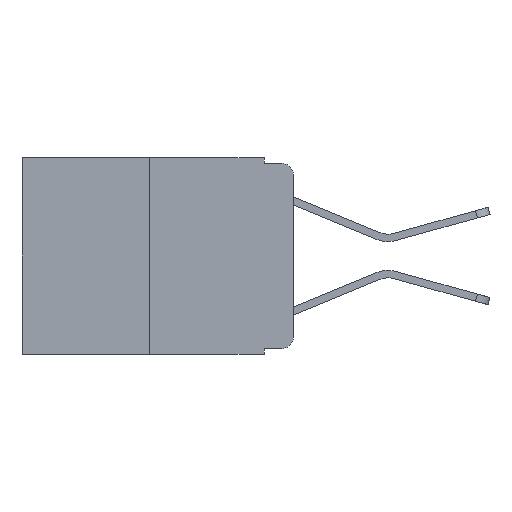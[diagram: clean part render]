
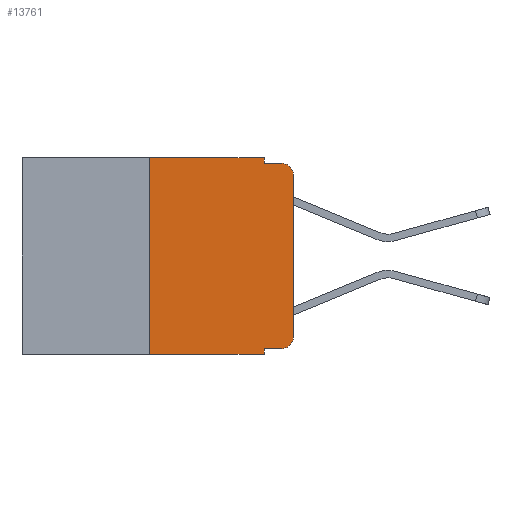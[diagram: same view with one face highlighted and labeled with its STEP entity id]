
A CAD part, left-side view. The second image highlights one B-rep face of the part: STEP entity #13761.
In plain terms, the highlighted planar face has unit normal (-1, 0, 0).
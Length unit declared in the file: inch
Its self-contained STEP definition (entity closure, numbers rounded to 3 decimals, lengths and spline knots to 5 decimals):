
#338 = VERTEX_POINT ( 'NONE', #4138 ) ;
#346 = DIRECTION ( 'NONE',  ( 1., 0., 0. ) ) ;
#349 = DIRECTION ( 'NONE',  ( 0., 0., -1. ) ) ;
#640 = VERTEX_POINT ( 'NONE', #7915 ) ;
#742 = CARTESIAN_POINT ( 'NONE',  ( 0., 0.051, 0. ) ) ;
#946 = VECTOR ( 'NONE', #1736, 39.37008 ) ;
#1036 = DIRECTION ( 'NONE',  ( -1., 0., 0. ) ) ;
#1514 = ORIENTED_EDGE ( 'NONE', *, *, #11581, .F. ) ;
#1736 = DIRECTION ( 'NONE',  ( 0., -1., 0. ) ) ;
#2160 = AXIS2_PLACEMENT_3D ( 'NONE', #17312, #9170, #349 ) ;
#2441 = ORIENTED_EDGE ( 'NONE', *, *, #17806, .F. ) ;
#2626 = LINE ( 'NONE', #14150, #10769 ) ;
#2885 = CARTESIAN_POINT ( 'NONE',  ( 0., 0.25, 0. ) ) ;
#2997 = CIRCLE ( 'NONE', #15039, 0.02 ) ;
#3247 = DIRECTION ( 'NONE',  ( 0., 0., 1. ) ) ;
#3428 = VECTOR ( 'NONE', #4094, 39.37008 ) ;
#3543 = DIRECTION ( 'NONE',  ( 0., 0., -1. ) ) ;
#4094 = DIRECTION ( 'NONE',  ( 0., 0., 1. ) ) ;
#4138 = CARTESIAN_POINT ( 'NONE',  ( 0., 0.02, -0.333 ) ) ;
#4234 = LINE ( 'NONE', #14015, #15026 ) ;
#4665 = AXIS2_PLACEMENT_3D ( 'NONE', #9167, #346, #10566 ) ;
#5112 = LINE ( 'NONE', #17452, #8095 ) ;
#5342 = DIRECTION ( 'NONE',  ( 0., -1., 0. ) ) ;
#5730 = DIRECTION ( 'NONE',  ( 0., 0., -1. ) ) ;
#5823 = LINE ( 'NONE', #17188, #17304 ) ;
#5868 = EDGE_CURVE ( 'NONE', #338, #16558, #2997, .T. ) ;
#6133 = CARTESIAN_POINT ( 'NONE',  ( 0., 0., -0.03 ) ) ;
#6172 = VERTEX_POINT ( 'NONE', #6133 ) ;
#6791 = ORIENTED_EDGE ( 'NONE', *, *, #9722, .F. ) ;
#6834 = EDGE_CURVE ( 'NONE', #640, #338, #14729, .T. ) ;
#6932 = EDGE_LOOP ( 'NONE', ( #8412, #12504, #1514, #13377, #2441, #6791, #10597, #11007, #14686, #11454 ) ) ;
#7082 = FACE_OUTER_BOUND ( 'NONE', #6932, .T. ) ;
#7103 = VERTEX_POINT ( 'NONE', #15554 ) ;
#7323 = LINE ( 'NONE', #12598, #3428 ) ;
#7479 = VERTEX_POINT ( 'NONE', #2885 ) ;
#7915 = CARTESIAN_POINT ( 'NONE',  ( 0., 0.051, -0.333 ) ) ;
#8095 = VECTOR ( 'NONE', #3543, 39.37008 ) ;
#8342 = LINE ( 'NONE', #10417, #946 ) ;
#8412 = ORIENTED_EDGE ( 'NONE', *, *, #13422, .T. ) ;
#8497 = CIRCLE ( 'NONE', #2160, 0.02 ) ;
#8804 = EDGE_CURVE ( 'NONE', #640, #11509, #2626, .T. ) ;
#9085 = CARTESIAN_POINT ( 'NONE',  ( 0., 0.25, -0.343 ) ) ;
#9167 = CARTESIAN_POINT ( 'NONE',  ( 0., 0.473, 0. ) ) ;
#9170 = DIRECTION ( 'NONE',  ( -1., 0., 0. ) ) ;
#9722 = EDGE_CURVE ( 'NONE', #14475, #7479, #5823, .T. ) ;
#9793 = CARTESIAN_POINT ( 'NONE',  ( 0., 0.02, -0.313 ) ) ;
#10417 = CARTESIAN_POINT ( 'NONE',  ( 0., 0.473, 0. ) ) ;
#10566 = DIRECTION ( 'NONE',  ( 0., 0., -1. ) ) ;
#10597 = ORIENTED_EDGE ( 'NONE', *, *, #17569, .T. ) ;
#10663 = EDGE_CURVE ( 'NONE', #13917, #13712, #5112, .T. ) ;
#10688 = LINE ( 'NONE', #14187, #17450 ) ;
#10769 = VECTOR ( 'NONE', #5730, 39.37008 ) ;
#11007 = ORIENTED_EDGE ( 'NONE', *, *, #8804, .F. ) ;
#11169 = DIRECTION ( 'NONE',  ( 0., 0., -1. ) ) ;
#11454 = ORIENTED_EDGE ( 'NONE', *, *, #5868, .T. ) ;
#11509 = VERTEX_POINT ( 'NONE', #14062 ) ;
#11581 = EDGE_CURVE ( 'NONE', #13712, #7103, #10688, .T. ) ;
#11824 = CARTESIAN_POINT ( 'NONE',  ( 0., 0.051, -0.01 ) ) ;
#12185 = CARTESIAN_POINT ( 'NONE',  ( 0., 0., -0.313 ) ) ;
#12482 = EDGE_CURVE ( 'NONE', #6172, #7103, #8497, .T. ) ;
#12504 = ORIENTED_EDGE ( 'NONE', *, *, #12482, .T. ) ;
#12598 = CARTESIAN_POINT ( 'NONE',  ( 0., 0., 0. ) ) ;
#13377 = ORIENTED_EDGE ( 'NONE', *, *, #10663, .F. ) ;
#13422 = EDGE_CURVE ( 'NONE', #16558, #6172, #7323, .T. ) ;
#13712 = VERTEX_POINT ( 'NONE', #11824 ) ;
#13761 = ADVANCED_FACE ( 'NONE', ( #7082 ), #17309, .F. ) ;
#13917 = VERTEX_POINT ( 'NONE', #742 ) ;
#14015 = CARTESIAN_POINT ( 'NONE',  ( 0., 0.473, -0.343 ) ) ;
#14062 = CARTESIAN_POINT ( 'NONE',  ( 0., 0.051, -0.343 ) ) ;
#14150 = CARTESIAN_POINT ( 'NONE',  ( 0., 0.051, 0. ) ) ;
#14187 = CARTESIAN_POINT ( 'NONE',  ( 0., 0.051, -0.01 ) ) ;
#14291 = VECTOR ( 'NONE', #5342, 39.37008 ) ;
#14475 = VERTEX_POINT ( 'NONE', #9085 ) ;
#14686 = ORIENTED_EDGE ( 'NONE', *, *, #6834, .T. ) ;
#14729 = LINE ( 'NONE', #17754, #14291 ) ;
#15026 = VECTOR ( 'NONE', #15384, 39.37008 ) ;
#15039 = AXIS2_PLACEMENT_3D ( 'NONE', #9793, #1036, #11169 ) ;
#15384 = DIRECTION ( 'NONE',  ( 0., -1., 0. ) ) ;
#15531 = DIRECTION ( 'NONE',  ( 0., -1., 0. ) ) ;
#15554 = CARTESIAN_POINT ( 'NONE',  ( 0., 0.02, -0.01 ) ) ;
#16558 = VERTEX_POINT ( 'NONE', #12185 ) ;
#17188 = CARTESIAN_POINT ( 'NONE',  ( 0., 0.25, 0. ) ) ;
#17304 = VECTOR ( 'NONE', #3247, 39.37008 ) ;
#17309 = PLANE ( 'NONE',  #4665 ) ;
#17312 = CARTESIAN_POINT ( 'NONE',  ( 0., 0.02, -0.03 ) ) ;
#17450 = VECTOR ( 'NONE', #15531, 39.37008 ) ;
#17452 = CARTESIAN_POINT ( 'NONE',  ( 0., 0.051, 0. ) ) ;
#17569 = EDGE_CURVE ( 'NONE', #14475, #11509, #4234, .T. ) ;
#17754 = CARTESIAN_POINT ( 'NONE',  ( 0., 0.051, -0.333 ) ) ;
#17806 = EDGE_CURVE ( 'NONE', #7479, #13917, #8342, .T. ) ;
